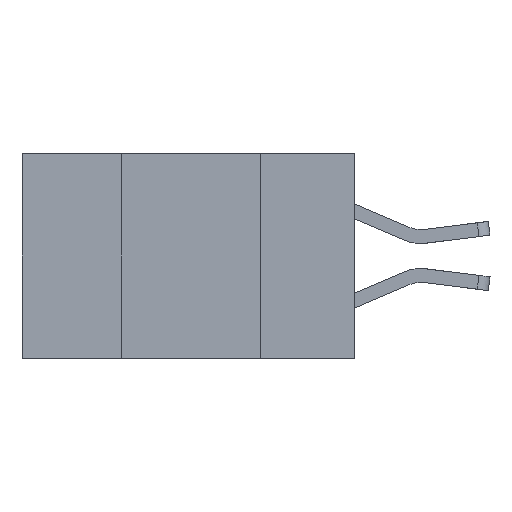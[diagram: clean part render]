
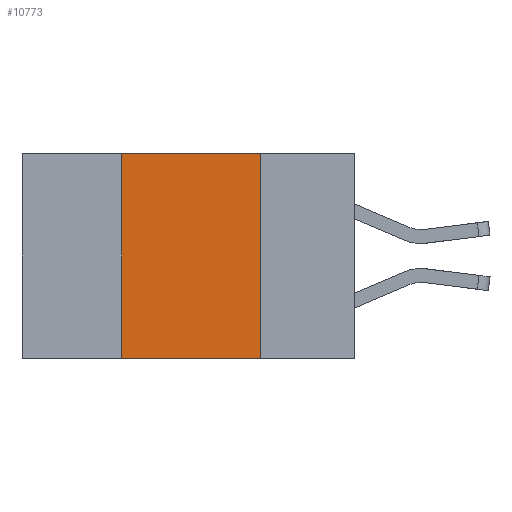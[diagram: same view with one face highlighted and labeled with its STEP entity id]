
A CAD part, left-side view. The second image highlights one B-rep face of the part: STEP entity #10773.
In plain terms, the highlighted planar face has unit normal (-1, 0, 0).
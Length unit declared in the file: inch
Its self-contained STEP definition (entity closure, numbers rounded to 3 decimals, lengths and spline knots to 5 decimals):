
#279 = VERTEX_POINT ( 'NONE', #1867 ) ;
#664 = VECTOR ( 'NONE', #5568, 39.37008 ) ;
#952 = ORIENTED_EDGE ( 'NONE', *, *, #4125, .F. ) ;
#1146 = VERTEX_POINT ( 'NONE', #7668 ) ;
#1220 = LINE ( 'NONE', #1471, #664 ) ;
#1373 = ORIENTED_EDGE ( 'NONE', *, *, #5106, .F. ) ;
#1471 = CARTESIAN_POINT ( 'NONE',  ( 0., 0.6, 0. ) ) ;
#1475 = CARTESIAN_POINT ( 'NONE',  ( 0., 0.42, 0. ) ) ;
#1499 = EDGE_CURVE ( 'NONE', #279, #1146, #9779, .T. ) ;
#1632 = VERTEX_POINT ( 'NONE', #6946 ) ;
#1867 = CARTESIAN_POINT ( 'NONE',  ( 0., 0.42, -0.37 ) ) ;
#2034 = DIRECTION ( 'NONE',  ( 1., 0., 0. ) ) ;
#2066 = EDGE_LOOP ( 'NONE', ( #952, #1373, #4044, #9817 ) ) ;
#2158 = VECTOR ( 'NONE', #6278, 39.37008 ) ;
#3049 = CARTESIAN_POINT ( 'NONE',  ( 0., 0.6, -0.37 ) ) ;
#4044 = ORIENTED_EDGE ( 'NONE', *, *, #1499, .F. ) ;
#4125 = EDGE_CURVE ( 'NONE', #10375, #1632, #5471, .T. ) ;
#4621 = VECTOR ( 'NONE', #9959, 39.37008 ) ;
#4706 = PLANE ( 'NONE',  #8085 ) ;
#5106 = EDGE_CURVE ( 'NONE', #1146, #10375, #1220, .T. ) ;
#5471 = LINE ( 'NONE', #10516, #2158 ) ;
#5568 = DIRECTION ( 'NONE',  ( 0., -1., 0. ) ) ;
#6083 = CARTESIAN_POINT ( 'NONE',  ( 0., 0.6, 0. ) ) ;
#6278 = DIRECTION ( 'NONE',  ( 0., 0., -1. ) ) ;
#6946 = CARTESIAN_POINT ( 'NONE',  ( 0., 0.17, -0.37 ) ) ;
#7149 = FACE_OUTER_BOUND ( 'NONE', #2066, .T. ) ;
#7153 = LINE ( 'NONE', #3049, #4621 ) ;
#7668 = CARTESIAN_POINT ( 'NONE',  ( 0., 0.42, 0. ) ) ;
#7732 = EDGE_CURVE ( 'NONE', #279, #1632, #7153, .T. ) ;
#8085 = AXIS2_PLACEMENT_3D ( 'NONE', #6083, #2034, #9308 ) ;
#8286 = VECTOR ( 'NONE', #9953, 39.37008 ) ;
#9308 = DIRECTION ( 'NONE',  ( 0., 0., -1. ) ) ;
#9779 = LINE ( 'NONE', #1475, #8286 ) ;
#9817 = ORIENTED_EDGE ( 'NONE', *, *, #7732, .T. ) ;
#9953 = DIRECTION ( 'NONE',  ( 0., 0., 1. ) ) ;
#9959 = DIRECTION ( 'NONE',  ( 0., -1., 0. ) ) ;
#10270 = CARTESIAN_POINT ( 'NONE',  ( 0., 0.17, 0. ) ) ;
#10375 = VERTEX_POINT ( 'NONE', #10270 ) ;
#10516 = CARTESIAN_POINT ( 'NONE',  ( 0., 0.17, 0. ) ) ;
#10773 = ADVANCED_FACE ( 'NONE', ( #7149 ), #4706, .F. ) ;
